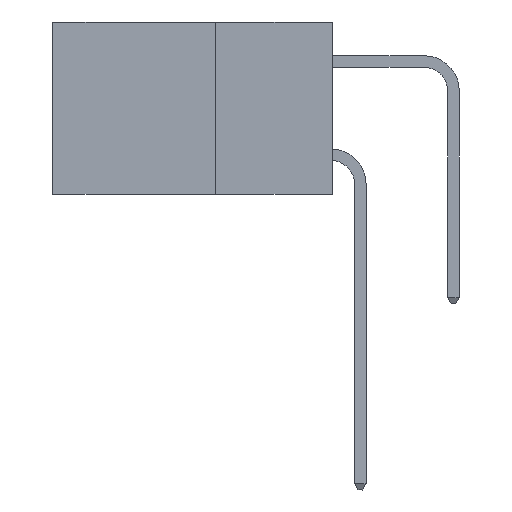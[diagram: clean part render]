
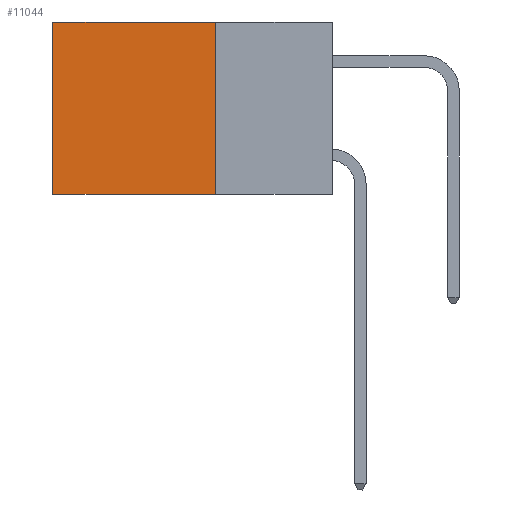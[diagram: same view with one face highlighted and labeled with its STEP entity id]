
A CAD part, left-side view. The second image highlights one B-rep face of the part: STEP entity #11044.
In plain terms, the highlighted planar face has unit normal (-1, 0, 0).
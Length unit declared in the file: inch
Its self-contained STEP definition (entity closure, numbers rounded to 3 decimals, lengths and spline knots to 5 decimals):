
#11 = DIRECTION ( 'NONE',  ( 1., 0., 0. ) ) ;
#162 = VECTOR ( 'NONE', #8115, 39.37008 ) ;
#1242 = CARTESIAN_POINT ( 'NONE',  ( 0.298, 0.25, 0. ) ) ;
#1379 = VERTEX_POINT ( 'NONE', #1398 ) ;
#1398 = CARTESIAN_POINT ( 'NONE',  ( 0.298, 0.6, -0.37 ) ) ;
#1634 = VERTEX_POINT ( 'NONE', #7472 ) ;
#2388 = DIRECTION ( 'NONE',  ( 0., 1., 0. ) ) ;
#2489 = DIRECTION ( 'NONE',  ( 0., 0., -1. ) ) ;
#4017 = EDGE_CURVE ( 'NONE', #1634, #12105, #11352, .T. ) ;
#4796 = VECTOR ( 'NONE', #2388, 39.37008 ) ;
#5728 = PLANE ( 'NONE',  #10495 ) ;
#5866 = VECTOR ( 'NONE', #2489, 39.37008 ) ;
#6150 = ORIENTED_EDGE ( 'NONE', *, *, #8265, .T. ) ;
#6291 = FACE_OUTER_BOUND ( 'NONE', #7114, .T. ) ;
#7114 = EDGE_LOOP ( 'NONE', ( #8859, #10088, #9040, #6150 ) ) ;
#7432 = CARTESIAN_POINT ( 'NONE',  ( 0.298, 0.25, -0.37 ) ) ;
#7472 = CARTESIAN_POINT ( 'NONE',  ( 0.298, 0.25, 0. ) ) ;
#7778 = CARTESIAN_POINT ( 'NONE',  ( 0.298, 0.25, -0.37 ) ) ;
#8054 = DIRECTION ( 'NONE',  ( 0., 0., -1. ) ) ;
#8072 = CARTESIAN_POINT ( 'NONE',  ( 0.298, 0.25, 0. ) ) ;
#8115 = DIRECTION ( 'NONE',  ( 0., 0., -1. ) ) ;
#8252 = VERTEX_POINT ( 'NONE', #13989 ) ;
#8265 = EDGE_CURVE ( 'NONE', #1634, #8252, #14073, .T. ) ;
#8586 = LINE ( 'NONE', #10619, #5866 ) ;
#8624 = DIRECTION ( 'NONE',  ( 0., 1., 0. ) ) ;
#8859 = ORIENTED_EDGE ( 'NONE', *, *, #14580, .T. ) ;
#9040 = ORIENTED_EDGE ( 'NONE', *, *, #4017, .F. ) ;
#9385 = LINE ( 'NONE', #7432, #11703 ) ;
#10088 = ORIENTED_EDGE ( 'NONE', *, *, #14122, .F. ) ;
#10495 = AXIS2_PLACEMENT_3D ( 'NONE', #13897, #11, #8054 ) ;
#10619 = CARTESIAN_POINT ( 'NONE',  ( 0.298, 0.6, 0. ) ) ;
#11044 = ADVANCED_FACE ( 'NONE', ( #6291 ), #5728, .F. ) ;
#11352 = LINE ( 'NONE', #8072, #162 ) ;
#11703 = VECTOR ( 'NONE', #8624, 39.37008 ) ;
#12105 = VERTEX_POINT ( 'NONE', #7778 ) ;
#13897 = CARTESIAN_POINT ( 'NONE',  ( 0.298, 0.25, 0. ) ) ;
#13989 = CARTESIAN_POINT ( 'NONE',  ( 0.298, 0.6, 0. ) ) ;
#14073 = LINE ( 'NONE', #1242, #4796 ) ;
#14122 = EDGE_CURVE ( 'NONE', #12105, #1379, #9385, .T. ) ;
#14580 = EDGE_CURVE ( 'NONE', #8252, #1379, #8586, .T. ) ;
